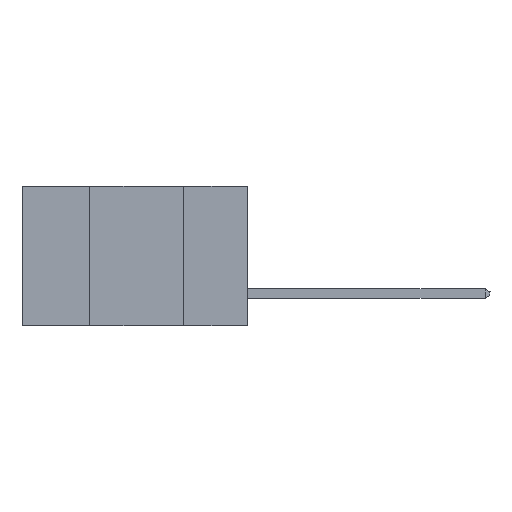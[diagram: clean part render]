
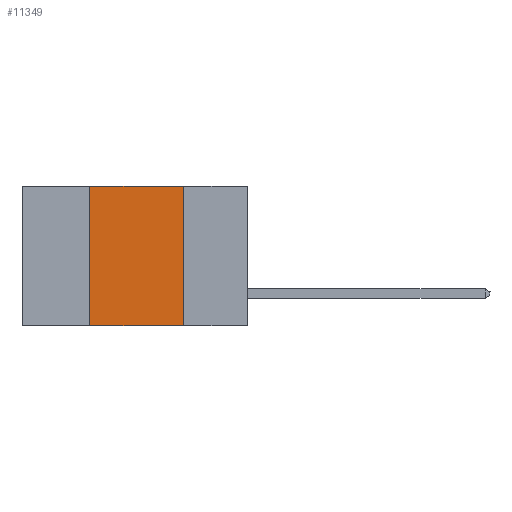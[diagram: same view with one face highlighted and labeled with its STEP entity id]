
A CAD part, left-side view. The second image highlights one B-rep face of the part: STEP entity #11349.
In plain terms, the highlighted planar face has unit normal (-1, 0, 0).
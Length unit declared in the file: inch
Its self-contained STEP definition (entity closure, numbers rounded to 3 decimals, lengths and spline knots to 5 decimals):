
#572 = FACE_OUTER_BOUND ( 'NONE', #16815, .T. ) ;
#634 = VECTOR ( 'NONE', #11762, 39.37008 ) ;
#967 = VERTEX_POINT ( 'NONE', #7363 ) ;
#1435 = EDGE_CURVE ( 'NONE', #8273, #8331, #5969, .T. ) ;
#1679 = DIRECTION ( 'NONE',  ( 0., 0., -1. ) ) ;
#3183 = AXIS2_PLACEMENT_3D ( 'NONE', #6163, #17356, #4786 ) ;
#4786 = DIRECTION ( 'NONE',  ( 0., 0., -1. ) ) ;
#4976 = LINE ( 'NONE', #7650, #634 ) ;
#5412 = LINE ( 'NONE', #8455, #12224 ) ;
#5969 = LINE ( 'NONE', #11550, #10526 ) ;
#6087 = CARTESIAN_POINT ( 'NONE',  ( 0., 0.17, -0.37 ) ) ;
#6163 = CARTESIAN_POINT ( 'NONE',  ( 0., 0.6, 0. ) ) ;
#7363 = CARTESIAN_POINT ( 'NONE',  ( 0., 0.42, 0. ) ) ;
#7456 = LINE ( 'NONE', #13054, #14172 ) ;
#7650 = CARTESIAN_POINT ( 'NONE',  ( 0., 0.6, 0. ) ) ;
#8248 = ORIENTED_EDGE ( 'NONE', *, *, #1435, .T. ) ;
#8273 = VERTEX_POINT ( 'NONE', #11586 ) ;
#8331 = VERTEX_POINT ( 'NONE', #6087 ) ;
#8455 = CARTESIAN_POINT ( 'NONE',  ( 0., 0.42, -0.37 ) ) ;
#10294 = EDGE_CURVE ( 'NONE', #8273, #967, #5412, .T. ) ;
#10526 = VECTOR ( 'NONE', #13119, 39.37008 ) ;
#10639 = ORIENTED_EDGE ( 'NONE', *, *, #15407, .F. ) ;
#11349 = ADVANCED_FACE ( 'NONE', ( #572 ), #15886, .F. ) ;
#11550 = CARTESIAN_POINT ( 'NONE',  ( 0., 0.6, -0.37 ) ) ;
#11586 = CARTESIAN_POINT ( 'NONE',  ( 0., 0.42, -0.37 ) ) ;
#11762 = DIRECTION ( 'NONE',  ( 0., -1., 0. ) ) ;
#12224 = VECTOR ( 'NONE', #15316, 39.37008 ) ;
#12302 = ORIENTED_EDGE ( 'NONE', *, *, #17826, .F. ) ;
#13054 = CARTESIAN_POINT ( 'NONE',  ( 0., 0.17, -0.37 ) ) ;
#13119 = DIRECTION ( 'NONE',  ( 0., -1., 0. ) ) ;
#14172 = VECTOR ( 'NONE', #1679, 39.37008 ) ;
#15316 = DIRECTION ( 'NONE',  ( 0., 0., 1. ) ) ;
#15407 = EDGE_CURVE ( 'NONE', #967, #15585, #4976, .T. ) ;
#15585 = VERTEX_POINT ( 'NONE', #17824 ) ;
#15886 = PLANE ( 'NONE',  #3183 ) ;
#16720 = ORIENTED_EDGE ( 'NONE', *, *, #10294, .F. ) ;
#16815 = EDGE_LOOP ( 'NONE', ( #12302, #10639, #16720, #8248 ) ) ;
#17356 = DIRECTION ( 'NONE',  ( 1., 0., 0. ) ) ;
#17824 = CARTESIAN_POINT ( 'NONE',  ( 0., 0.17, 0. ) ) ;
#17826 = EDGE_CURVE ( 'NONE', #15585, #8331, #7456, .T. ) ;
